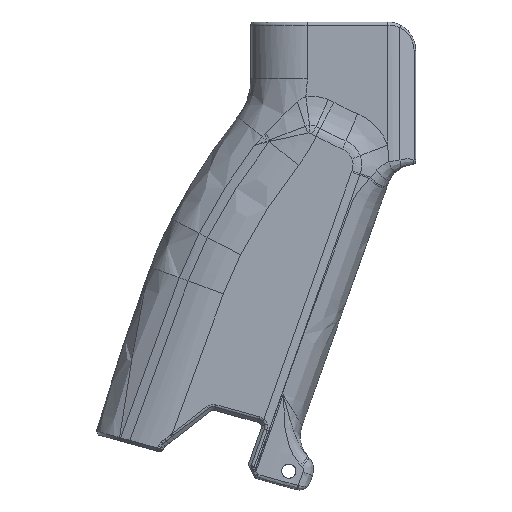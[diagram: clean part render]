
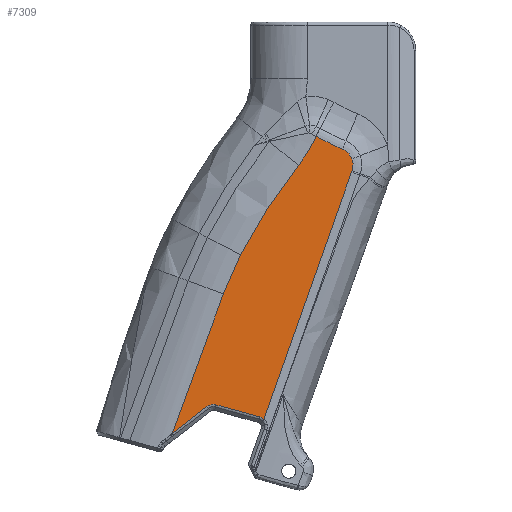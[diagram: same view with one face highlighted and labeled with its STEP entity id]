
A CAD part, left-side view. The second image highlights one B-rep face of the part: STEP entity #7309.
In plain terms, the highlighted planar face has unit normal (-1, 0, 0).
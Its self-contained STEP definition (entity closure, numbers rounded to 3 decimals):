
#588=CIRCLE('',#7751,2.311);
#594=CIRCLE('',#7759,2.311);
#607=CIRCLE('',#7790,3.889);
#608=CIRCLE('',#7791,75.936);
#1003=FACE_OUTER_BOUND('',#1476,.T.);
#1476=EDGE_LOOP('',(#6133,#6134,#6135,#6136,#6137,#6138,#6139,#6140,#6141,
#6142,#6143,#6144,#6145));
#2046=B_SPLINE_CURVE_WITH_KNOTS('',3,(#17749,#17750,#17751,#17752),
 .UNSPECIFIED.,.F.,.F.,(4,4),(-0.031,0.),
 .UNSPECIFIED.);
#2047=B_SPLINE_CURVE_WITH_KNOTS('',3,(#17754,#17755,#17756,#17757),
 .UNSPECIFIED.,.F.,.F.,(4,4),(0.,0.275),.UNSPECIFIED.);
#2048=B_SPLINE_CURVE_WITH_KNOTS('',3,(#17763,#17764,#17765,#17766),
 .UNSPECIFIED.,.F.,.F.,(4,4),(-0.596,0.166),
 .UNSPECIFIED.);
#2049=B_SPLINE_CURVE_WITH_KNOTS('',3,(#17768,#17769,#17770,#17771),
 .UNSPECIFIED.,.F.,.F.,(4,4),(-2.413,0.),.UNSPECIFIED.);
#2050=B_SPLINE_CURVE_WITH_KNOTS('',3,(#17772,#17773,#17774,#17775),
 .UNSPECIFIED.,.F.,.F.,(4,4),(-0.965,0.),.UNSPECIFIED.);
#2227=LINE('',#10463,#2521);
#2414=LINE('',#17349,#2708);
#2416=LINE('',#17361,#2710);
#2429=LINE('',#17640,#2723);
#2521=VECTOR('',#8024,10.);
#2708=VECTOR('',#8693,10.);
#2710=VECTOR('',#8707,10.);
#2723=VECTOR('',#8746,10.);
#2868=VERTEX_POINT('',#10460);
#2869=VERTEX_POINT('',#10462);
#3274=VERTEX_POINT('',#17339);
#3276=VERTEX_POINT('',#17345);
#3278=VERTEX_POINT('',#17351);
#3280=VERTEX_POINT('',#17357);
#3299=VERTEX_POINT('',#17639);
#3312=VERTEX_POINT('',#17748);
#3313=VERTEX_POINT('',#17753);
#3314=VERTEX_POINT('',#17758);
#3315=VERTEX_POINT('',#17760);
#3316=VERTEX_POINT('',#17762);
#3317=VERTEX_POINT('',#17767);
#3573=EDGE_CURVE('',#2868,#2869,#2227,.T.);
#4227=EDGE_CURVE('',#2869,#3274,#588,.T.);
#4232=EDGE_CURVE('',#3274,#3276,#2414,.T.);
#4235=EDGE_CURVE('',#3276,#3278,#594,.T.);
#4238=EDGE_CURVE('',#3278,#3280,#2416,.T.);
#4272=EDGE_CURVE('',#3280,#3299,#2429,.T.);
#4296=EDGE_CURVE('',#3312,#2868,#2046,.T.);
#4297=EDGE_CURVE('',#3313,#3312,#2047,.T.);
#4298=EDGE_CURVE('',#3314,#3313,#607,.T.);
#4299=EDGE_CURVE('',#3315,#3314,#608,.T.);
#4300=EDGE_CURVE('',#3316,#3315,#2048,.T.);
#4301=EDGE_CURVE('',#3317,#3316,#2049,.T.);
#4302=EDGE_CURVE('',#3299,#3317,#2050,.T.);
#6133=ORIENTED_EDGE('',*,*,#4227,.F.);
#6134=ORIENTED_EDGE('',*,*,#3573,.F.);
#6135=ORIENTED_EDGE('',*,*,#4296,.F.);
#6136=ORIENTED_EDGE('',*,*,#4297,.F.);
#6137=ORIENTED_EDGE('',*,*,#4298,.F.);
#6138=ORIENTED_EDGE('',*,*,#4299,.F.);
#6139=ORIENTED_EDGE('',*,*,#4300,.F.);
#6140=ORIENTED_EDGE('',*,*,#4301,.F.);
#6141=ORIENTED_EDGE('',*,*,#4302,.F.);
#6142=ORIENTED_EDGE('',*,*,#4272,.F.);
#6143=ORIENTED_EDGE('',*,*,#4238,.F.);
#6144=ORIENTED_EDGE('',*,*,#4235,.F.);
#6145=ORIENTED_EDGE('',*,*,#4232,.F.);
#6980=PLANE('',#7789);
#7309=ADVANCED_FACE('',(#1003),#6980,.T.);
#7751=AXIS2_PLACEMENT_3D('',#17340,#8682,#8683);
#7759=AXIS2_PLACEMENT_3D('',#17355,#8700,#8701);
#7789=AXIS2_PLACEMENT_3D('',#17747,#8785,#8786);
#7790=AXIS2_PLACEMENT_3D('',#17759,#8787,#8788);
#7791=AXIS2_PLACEMENT_3D('',#17761,#8789,#8790);
#8024=DIRECTION('',(0.,0.335,-0.942));
#8682=DIRECTION('center_axis',(-1.,0.,0.));
#8683=DIRECTION('ref_axis',(0.,-0.499,0.867));
#8693=DIRECTION('',(0.,0.964,0.266));
#8700=DIRECTION('center_axis',(-1.,0.,0.));
#8701=DIRECTION('ref_axis',(0.,0.194,0.981));
#8707=DIRECTION('',(0.,0.79,-0.613));
#8746=DIRECTION('',(0.,-0.344,0.939));
#8785=DIRECTION('center_axis',(-1.,0.,0.));
#8786=DIRECTION('ref_axis',(0.,-1.,0.));
#8787=DIRECTION('center_axis',(1.,0.,0.));
#8788=DIRECTION('ref_axis',(0.,-0.72,0.694));
#8789=DIRECTION('center_axis',(-1.,0.,0.));
#8790=DIRECTION('ref_axis',(0.,0.433,-0.901));
#10460=CARTESIAN_POINT('',(-13.29,-139.811,-43.074));
#10462=CARTESIAN_POINT('',(-13.29,-119.985,-98.836));
#10463=CARTESIAN_POINT('',(-13.29,-123.761,-88.216));
#17339=CARTESIAN_POINT('',(-13.29,-119.086,-98.354));
#17340=CARTESIAN_POINT('Origin',(-13.29,-118.471,-100.581));
#17345=CARTESIAN_POINT('',(-13.29,-109.196,-95.624));
#17349=CARTESIAN_POINT('',(-13.29,-111.571,-96.279));
#17351=CARTESIAN_POINT('',(-13.29,-107.164,-96.026));
#17355=CARTESIAN_POINT('Origin',(-13.29,-108.581,-97.851));
#17357=CARTESIAN_POINT('',(-13.29,-99.336,-102.103));
#17361=CARTESIAN_POINT('',(-13.29,-126.252,-81.205));
#17639=CARTESIAN_POINT('',(-13.29,-110.892,-70.588));
#17640=CARTESIAN_POINT('',(-13.29,-110.892,-70.588));
#17747=CARTESIAN_POINT('Origin',(-13.29,-121.21,-61.501));
#17748=CARTESIAN_POINT('',(-13.29,-139.915,-42.781));
#17749=CARTESIAN_POINT('Ctrl Pts',(-13.29,-139.915,
-42.781));
#17750=CARTESIAN_POINT('Ctrl Pts',(-13.29,-139.88,
-42.879));
#17751=CARTESIAN_POINT('Ctrl Pts',(-13.29,-139.845,
-42.977));
#17752=CARTESIAN_POINT('Ctrl Pts',(-13.29,-139.811,
-43.074));
#17753=CARTESIAN_POINT('',(-13.29,-139.883,-40.083));
#17754=CARTESIAN_POINT('Ctrl Pts',(-13.29,-139.883,-40.083));
#17755=CARTESIAN_POINT('Ctrl Pts',(-13.29,-140.212,
-40.94));
#17756=CARTESIAN_POINT('Ctrl Pts',(-13.29,-140.222,
-41.916));
#17757=CARTESIAN_POINT('Ctrl Pts',(-13.29,-139.915,
-42.781));
#17758=CARTESIAN_POINT('',(-13.29,-137.78,-37.898));
#17759=CARTESIAN_POINT('Origin',(-13.29,-136.252,-41.474));
#17760=CARTESIAN_POINT('',(-13.29,-131.81,-35.034));
#17761=CARTESIAN_POINT('Origin',(-13.29,-167.611,31.933));
#17762=CARTESIAN_POINT('',(-13.29,-127.852,-41.526));
#17763=CARTESIAN_POINT('Ctrl Pts',(-13.29,-127.852,
-41.526));
#17764=CARTESIAN_POINT('Ctrl Pts',(-13.29,-129.427,-39.533));
#17765=CARTESIAN_POINT('Ctrl Pts',(-13.29,-130.759,
-37.348));
#17766=CARTESIAN_POINT('Ctrl Pts',(-13.29,-131.81,
-35.034));
#17767=CARTESIAN_POINT('',(-13.29,-114.781,-61.762));
#17768=CARTESIAN_POINT('Ctrl Pts',(-13.29,-114.781,
-61.762));
#17769=CARTESIAN_POINT('Ctrl Pts',(-13.29,-118.484,
-54.623));
#17770=CARTESIAN_POINT('Ctrl Pts',(-13.29,-122.867,
-47.837));
#17771=CARTESIAN_POINT('Ctrl Pts',(-13.29,-127.852,
-41.526));
#17772=CARTESIAN_POINT('Ctrl Pts',(-13.29,-110.892,
-70.588));
#17773=CARTESIAN_POINT('Ctrl Pts',(-13.29,-111.999,
-67.568));
#17774=CARTESIAN_POINT('Ctrl Pts',(-13.29,-113.299,
-64.618));
#17775=CARTESIAN_POINT('Ctrl Pts',(-13.29,-114.781,
-61.762));
